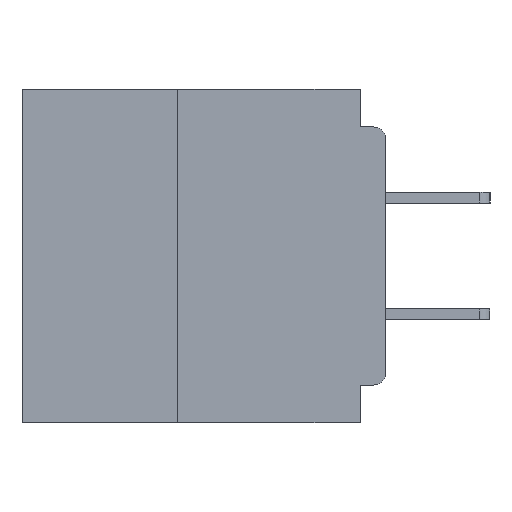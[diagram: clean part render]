
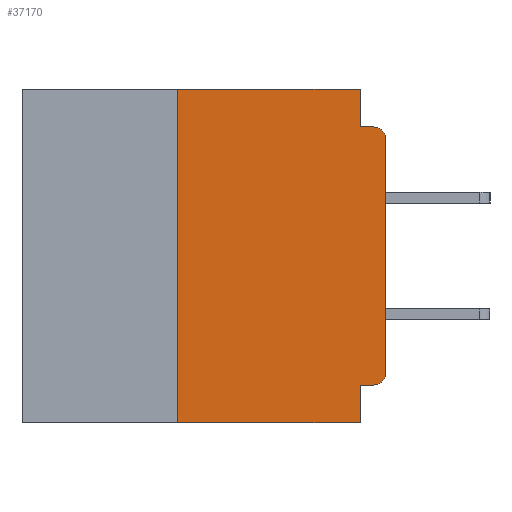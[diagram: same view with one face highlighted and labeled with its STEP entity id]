
A CAD part, left-side view. The second image highlights one B-rep face of the part: STEP entity #37170.
In plain terms, the highlighted planar face has unit normal (-1, 0, 0).
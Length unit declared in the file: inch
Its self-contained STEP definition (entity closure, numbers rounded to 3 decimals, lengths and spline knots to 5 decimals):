
#768 = ORIENTED_EDGE ( 'NONE', *, *, #9655, .F. ) ;
#859 = ORIENTED_EDGE ( 'NONE', *, *, #26902, .F. ) ;
#1425 = CIRCLE ( 'NONE', #27337, 0.015 ) ;
#1474 = FACE_OUTER_BOUND ( 'NONE', #43497, .T. ) ;
#1577 = VERTEX_POINT ( 'NONE', #6517 ) ;
#2102 = CARTESIAN_POINT ( 'NONE',  ( 0., 0.015, -0.34 ) ) ;
#3790 = EDGE_CURVE ( 'NONE', #15035, #33599, #8572, .T. ) ;
#3901 = DIRECTION ( 'NONE',  ( 0., 0., -1. ) ) ;
#4467 = VERTEX_POINT ( 'NONE', #15434 ) ;
#5099 = DIRECTION ( 'NONE',  ( 0., 1., 0. ) ) ;
#5368 = LINE ( 'NONE', #43220, #43848 ) ;
#5684 = EDGE_CURVE ( 'NONE', #16339, #47859, #48896, .T. ) ;
#5969 = DIRECTION ( 'NONE',  ( 0., 0., -1. ) ) ;
#6211 = CIRCLE ( 'NONE', #7244, 0.015 ) ;
#6517 = CARTESIAN_POINT ( 'NONE',  ( 0., 0., -0.06 ) ) ;
#7244 = AXIS2_PLACEMENT_3D ( 'NONE', #16512, #43230, #20403 ) ;
#7684 = CARTESIAN_POINT ( 'NONE',  ( 0., 0.031, -0.045 ) ) ;
#7823 = DIRECTION ( 'NONE',  ( 0., 0., 1. ) ) ;
#8104 = ORIENTED_EDGE ( 'NONE', *, *, #5684, .T. ) ;
#8135 = LINE ( 'NONE', #42153, #17311 ) ;
#8572 = LINE ( 'NONE', #32297, #39245 ) ;
#9465 = LINE ( 'NONE', #44205, #37712 ) ;
#9655 = EDGE_CURVE ( 'NONE', #37112, #15035, #5368, .T. ) ;
#10390 = DIRECTION ( 'NONE',  ( 0., 0., 1. ) ) ;
#11874 = ORIENTED_EDGE ( 'NONE', *, *, #30493, .T. ) ;
#13755 = DIRECTION ( 'NONE',  ( 0., -1., 0. ) ) ;
#13829 = CARTESIAN_POINT ( 'NONE',  ( 0., 0., -0.34 ) ) ;
#14056 = AXIS2_PLACEMENT_3D ( 'NONE', #46034, #27131, #3901 ) ;
#14062 = EDGE_CURVE ( 'NONE', #26002, #37112, #9465, .T. ) ;
#14183 = ORIENTED_EDGE ( 'NONE', *, *, #14062, .F. ) ;
#15035 = VERTEX_POINT ( 'NONE', #7684 ) ;
#15409 = LINE ( 'NONE', #42419, #44685 ) ;
#15434 = CARTESIAN_POINT ( 'NONE',  ( 0., 0.015, -0.355 ) ) ;
#15995 = LINE ( 'NONE', #32106, #45262 ) ;
#16339 = VERTEX_POINT ( 'NONE', #24061 ) ;
#16512 = CARTESIAN_POINT ( 'NONE',  ( 0., 0.015, -0.06 ) ) ;
#17311 = VECTOR ( 'NONE', #23201, 39.37008 ) ;
#17811 = ORIENTED_EDGE ( 'NONE', *, *, #3790, .F. ) ;
#18379 = CARTESIAN_POINT ( 'NONE',  ( 0., 0.031, -0.4 ) ) ;
#19151 = CARTESIAN_POINT ( 'NONE',  ( 0., 0.031, -0.355 ) ) ;
#19377 = PLANE ( 'NONE',  #14056 ) ;
#20403 = DIRECTION ( 'NONE',  ( 0., 0., -1. ) ) ;
#20632 = DIRECTION ( 'NONE',  ( 0., -1., 0. ) ) ;
#21029 = CARTESIAN_POINT ( 'NONE',  ( 0., 0.437, -0.4 ) ) ;
#23201 = DIRECTION ( 'NONE',  ( 0., 0., -1. ) ) ;
#24061 = CARTESIAN_POINT ( 'NONE',  ( 0., 0.25, -0.4 ) ) ;
#26002 = VERTEX_POINT ( 'NONE', #26456 ) ;
#26014 = VECTOR ( 'NONE', #10390, 39.37008 ) ;
#26456 = CARTESIAN_POINT ( 'NONE',  ( 0., 0.25, 0. ) ) ;
#26902 = EDGE_CURVE ( 'NONE', #37771, #47859, #8135, .T. ) ;
#27131 = DIRECTION ( 'NONE',  ( 1., 0., 0. ) ) ;
#27337 = AXIS2_PLACEMENT_3D ( 'NONE', #2102, #29138, #5969 ) ;
#27411 = ORIENTED_EDGE ( 'NONE', *, *, #30932, .T. ) ;
#27607 = EDGE_CURVE ( 'NONE', #30533, #1577, #15409, .T. ) ;
#27807 = EDGE_CURVE ( 'NONE', #4467, #37771, #15995, .T. ) ;
#28072 = CARTESIAN_POINT ( 'NONE',  ( 0., 0.015, -0.045 ) ) ;
#28108 = DIRECTION ( 'NONE',  ( 0., 0., -1. ) ) ;
#29138 = DIRECTION ( 'NONE',  ( -1., 0., 0. ) ) ;
#30493 = EDGE_CURVE ( 'NONE', #4467, #30533, #1425, .T. ) ;
#30533 = VERTEX_POINT ( 'NONE', #13829 ) ;
#30587 = CARTESIAN_POINT ( 'NONE',  ( 0., 0.031, 0. ) ) ;
#30932 = EDGE_CURVE ( 'NONE', #1577, #33599, #6211, .T. ) ;
#31676 = ORIENTED_EDGE ( 'NONE', *, *, #27807, .F. ) ;
#32106 = CARTESIAN_POINT ( 'NONE',  ( 0., 0., -0.355 ) ) ;
#32297 = CARTESIAN_POINT ( 'NONE',  ( 0., 0., -0.045 ) ) ;
#33112 = DIRECTION ( 'NONE',  ( 0., -1., 0. ) ) ;
#33599 = VERTEX_POINT ( 'NONE', #28072 ) ;
#35209 = ORIENTED_EDGE ( 'NONE', *, *, #40256, .F. ) ;
#36090 = LINE ( 'NONE', #37279, #26014 ) ;
#37112 = VERTEX_POINT ( 'NONE', #30587 ) ;
#37170 = ADVANCED_FACE ( 'NONE', ( #1474 ), #19377, .F. ) ;
#37279 = CARTESIAN_POINT ( 'NONE',  ( 0., 0.25, -0.4 ) ) ;
#37712 = VECTOR ( 'NONE', #13755, 39.37008 ) ;
#37771 = VERTEX_POINT ( 'NONE', #19151 ) ;
#38799 = VECTOR ( 'NONE', #20632, 39.37008 ) ;
#39245 = VECTOR ( 'NONE', #33112, 39.37008 ) ;
#40256 = EDGE_CURVE ( 'NONE', #16339, #26002, #36090, .T. ) ;
#42153 = CARTESIAN_POINT ( 'NONE',  ( 0., 0.031, -0.4 ) ) ;
#42419 = CARTESIAN_POINT ( 'NONE',  ( 0., 0., 0. ) ) ;
#43220 = CARTESIAN_POINT ( 'NONE',  ( 0., 0.031, 0. ) ) ;
#43230 = DIRECTION ( 'NONE',  ( -1., 0., 0. ) ) ;
#43497 = EDGE_LOOP ( 'NONE', ( #47555, #27411, #17811, #768, #14183, #35209, #8104, #859, #31676, #11874 ) ) ;
#43848 = VECTOR ( 'NONE', #28108, 39.37008 ) ;
#44205 = CARTESIAN_POINT ( 'NONE',  ( 0., 0.437, 0. ) ) ;
#44685 = VECTOR ( 'NONE', #7823, 39.37008 ) ;
#45262 = VECTOR ( 'NONE', #5099, 39.37008 ) ;
#46034 = CARTESIAN_POINT ( 'NONE',  ( 0., 0.437, 0. ) ) ;
#47555 = ORIENTED_EDGE ( 'NONE', *, *, #27607, .T. ) ;
#47859 = VERTEX_POINT ( 'NONE', #18379 ) ;
#48896 = LINE ( 'NONE', #21029, #38799 ) ;
